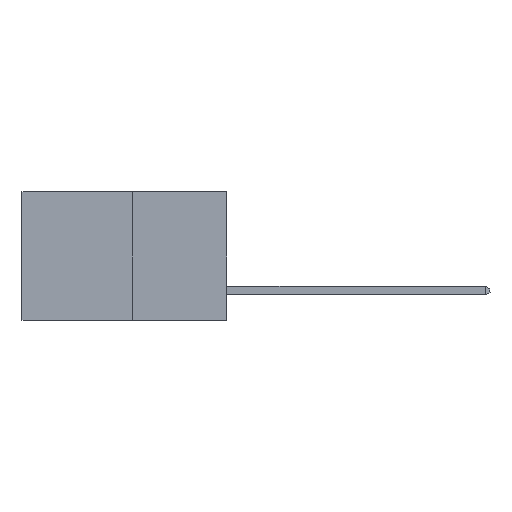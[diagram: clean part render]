
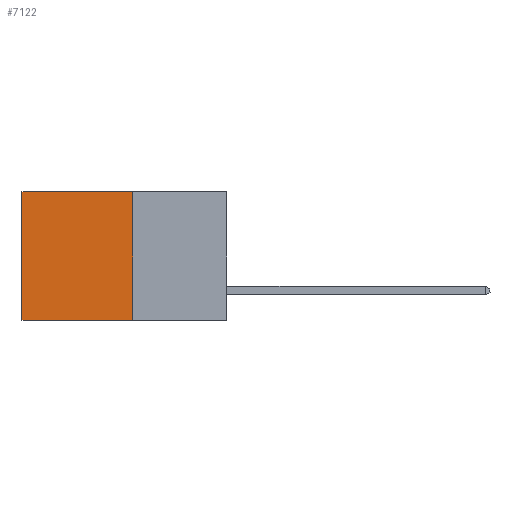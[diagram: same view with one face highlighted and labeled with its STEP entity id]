
A CAD part, left-side view. The second image highlights one B-rep face of the part: STEP entity #7122.
In plain terms, the highlighted planar face has unit normal (-1, 0, 0).
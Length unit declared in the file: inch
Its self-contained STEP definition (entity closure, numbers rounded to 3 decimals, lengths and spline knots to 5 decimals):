
#868 = VECTOR ( 'NONE', #1484, 39.37008 ) ;
#1097 = LINE ( 'NONE', #2957, #868 ) ;
#1279 = EDGE_CURVE ( 'NONE', #7981, #3709, #6825, .T. ) ;
#1484 = DIRECTION ( 'NONE',  ( 0., 0., -1. ) ) ;
#1946 = CARTESIAN_POINT ( 'NONE',  ( 0.277, 0.27, -0.37 ) ) ;
#2111 = FACE_OUTER_BOUND ( 'NONE', #2298, .T. ) ;
#2150 = CARTESIAN_POINT ( 'NONE',  ( 0.277, 0.59, 0. ) ) ;
#2298 = EDGE_LOOP ( 'NONE', ( #4598, #2936, #4794, #8302 ) ) ;
#2936 = ORIENTED_EDGE ( 'NONE', *, *, #1279, .F. ) ;
#2957 = CARTESIAN_POINT ( 'NONE',  ( 0.277, 0.27, -0.37 ) ) ;
#3023 = VECTOR ( 'NONE', #8032, 39.37008 ) ;
#3187 = VECTOR ( 'NONE', #6586, 39.37008 ) ;
#3394 = CARTESIAN_POINT ( 'NONE',  ( 0.277, 0.59, -0.37 ) ) ;
#3476 = CARTESIAN_POINT ( 'NONE',  ( 0.277, 0.59, -0.37 ) ) ;
#3709 = VERTEX_POINT ( 'NONE', #3476 ) ;
#3894 = VECTOR ( 'NONE', #5273, 39.37008 ) ;
#4170 = EDGE_CURVE ( 'NONE', #4443, #3709, #4672, .T. ) ;
#4443 = VERTEX_POINT ( 'NONE', #2150 ) ;
#4598 = ORIENTED_EDGE ( 'NONE', *, *, #4170, .T. ) ;
#4672 = LINE ( 'NONE', #3394, #3023 ) ;
#4794 = ORIENTED_EDGE ( 'NONE', *, *, #7512, .F. ) ;
#5240 = CARTESIAN_POINT ( 'NONE',  ( 0.277, 0.27, 0. ) ) ;
#5273 = DIRECTION ( 'NONE',  ( 0., 1., 0. ) ) ;
#5674 = LINE ( 'NONE', #5240, #3894 ) ;
#5726 = CARTESIAN_POINT ( 'NONE',  ( 0.277, 0.27, 0. ) ) ;
#6088 = VERTEX_POINT ( 'NONE', #5726 ) ;
#6127 = CARTESIAN_POINT ( 'NONE',  ( 0.277, 0.27, -0.37 ) ) ;
#6492 = EDGE_CURVE ( 'NONE', #6088, #4443, #5674, .T. ) ;
#6586 = DIRECTION ( 'NONE',  ( 0., 1., 0. ) ) ;
#6825 = LINE ( 'NONE', #6127, #3187 ) ;
#6991 = AXIS2_PLACEMENT_3D ( 'NONE', #7030, #8000, #7941 ) ;
#7030 = CARTESIAN_POINT ( 'NONE',  ( 0.277, 0.27, -0.37 ) ) ;
#7122 = ADVANCED_FACE ( 'NONE', ( #2111 ), #7842, .F. ) ;
#7512 = EDGE_CURVE ( 'NONE', #6088, #7981, #1097, .T. ) ;
#7842 = PLANE ( 'NONE',  #6991 ) ;
#7941 = DIRECTION ( 'NONE',  ( 0., 0., -1. ) ) ;
#7981 = VERTEX_POINT ( 'NONE', #1946 ) ;
#8000 = DIRECTION ( 'NONE',  ( 1., 0., 0. ) ) ;
#8032 = DIRECTION ( 'NONE',  ( 0., 0., -1. ) ) ;
#8302 = ORIENTED_EDGE ( 'NONE', *, *, #6492, .T. ) ;
